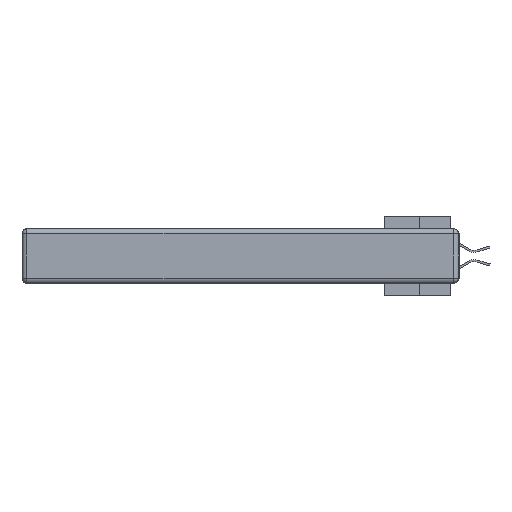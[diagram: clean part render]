
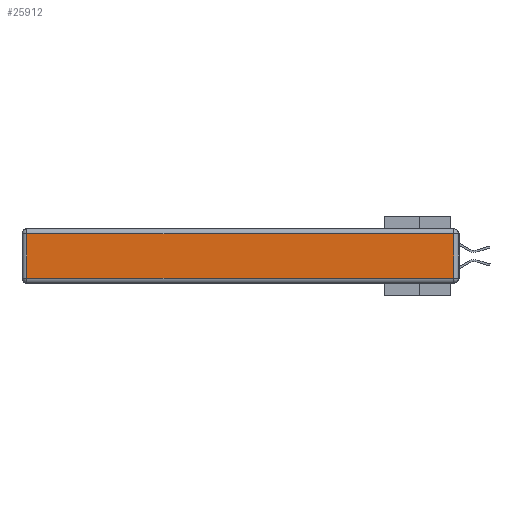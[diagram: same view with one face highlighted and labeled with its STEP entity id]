
A CAD part, left-side view. The second image highlights one B-rep face of the part: STEP entity #25912.
In plain terms, the highlighted planar face has unit normal (-1, 0, 0).
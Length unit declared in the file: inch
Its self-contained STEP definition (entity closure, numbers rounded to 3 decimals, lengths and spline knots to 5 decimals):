
#370 = ORIENTED_EDGE ( 'NONE', *, *, #15044, .T. ) ;
#633 = CARTESIAN_POINT ( 'NONE',  ( 0., 2.72, -0.343 ) ) ;
#2048 = CARTESIAN_POINT ( 'NONE',  ( 0., 0.03, -0.03 ) ) ;
#2267 = VERTEX_POINT ( 'NONE', #16256 ) ;
#2485 = AXIS2_PLACEMENT_3D ( 'NONE', #23451, #20857, #2691 ) ;
#2497 = FACE_OUTER_BOUND ( 'NONE', #7860, .T. ) ;
#2691 = DIRECTION ( 'NONE',  ( 0., 0., 1. ) ) ;
#3228 = LINE ( 'NONE', #633, #10167 ) ;
#4341 = ORIENTED_EDGE ( 'NONE', *, *, #26451, .T. ) ;
#7860 = EDGE_LOOP ( 'NONE', ( #13061, #370, #28153, #4341 ) ) ;
#10167 = VECTOR ( 'NONE', #36579, 39.37008 ) ;
#12305 = CARTESIAN_POINT ( 'NONE',  ( 0., 2.72, -0.03 ) ) ;
#12361 = LINE ( 'NONE', #34918, #23490 ) ;
#13061 = ORIENTED_EDGE ( 'NONE', *, *, #34002, .T. ) ;
#14693 = VERTEX_POINT ( 'NONE', #21893 ) ;
#15044 = EDGE_CURVE ( 'NONE', #14693, #25112, #34258, .T. ) ;
#16256 = CARTESIAN_POINT ( 'NONE',  ( 0., 2.72, -0.313 ) ) ;
#18260 = LINE ( 'NONE', #24436, #19700 ) ;
#19700 = VECTOR ( 'NONE', #36829, 39.37008 ) ;
#20857 = DIRECTION ( 'NONE',  ( -1., 0., 0. ) ) ;
#21498 = VECTOR ( 'NONE', #24851, 39.37008 ) ;
#21893 = CARTESIAN_POINT ( 'NONE',  ( 0., 0.03, -0.313 ) ) ;
#22052 = CARTESIAN_POINT ( 'NONE',  ( 0., 0.03, -0.343 ) ) ;
#23451 = CARTESIAN_POINT ( 'NONE',  ( 0., 0., -0.343 ) ) ;
#23490 = VECTOR ( 'NONE', #34526, 39.37008 ) ;
#24250 = VERTEX_POINT ( 'NONE', #12305 ) ;
#24436 = CARTESIAN_POINT ( 'NONE',  ( 0., 2.75, -0.03 ) ) ;
#24851 = DIRECTION ( 'NONE',  ( 0., 0., 1. ) ) ;
#25112 = VERTEX_POINT ( 'NONE', #2048 ) ;
#25912 = ADVANCED_FACE ( 'NONE', ( #2497 ), #29452, .T. ) ;
#26451 = EDGE_CURVE ( 'NONE', #24250, #2267, #3228, .T. ) ;
#28153 = ORIENTED_EDGE ( 'NONE', *, *, #36245, .T. ) ;
#29452 = PLANE ( 'NONE',  #2485 ) ;
#34002 = EDGE_CURVE ( 'NONE', #2267, #14693, #12361, .T. ) ;
#34258 = LINE ( 'NONE', #22052, #21498 ) ;
#34526 = DIRECTION ( 'NONE',  ( 0., -1., 0. ) ) ;
#34918 = CARTESIAN_POINT ( 'NONE',  ( 0., 0., -0.313 ) ) ;
#36245 = EDGE_CURVE ( 'NONE', #25112, #24250, #18260, .T. ) ;
#36579 = DIRECTION ( 'NONE',  ( 0., 0., -1. ) ) ;
#36829 = DIRECTION ( 'NONE',  ( 0., 1., 0. ) ) ;
